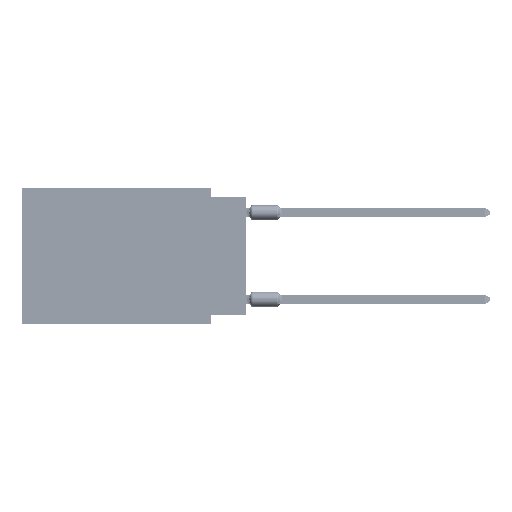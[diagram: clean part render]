
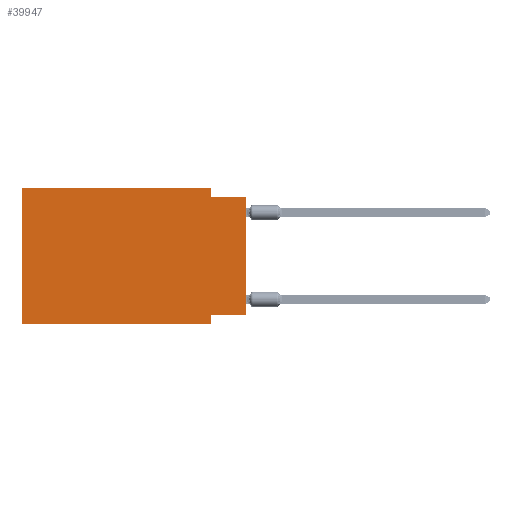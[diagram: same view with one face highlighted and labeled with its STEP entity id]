
A CAD part, left-side view. The second image highlights one B-rep face of the part: STEP entity #39947.
In plain terms, the highlighted planar face has unit normal (-1, 0, 0).
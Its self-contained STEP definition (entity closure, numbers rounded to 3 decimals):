
#1389 = ORIENTED_EDGE ( 'NONE', *, *, #11640, .F. ) ;
#4130 = ORIENTED_EDGE ( 'NONE', *, *, #25909, .F. ) ;
#4822 = CARTESIAN_POINT ( 'NONE',  ( 0., 16.383, 0. ) ) ;
#5756 = CARTESIAN_POINT ( 'NONE',  ( 0., 2.54, 0. ) ) ;
#6396 = DIRECTION ( 'NONE',  ( 0., 0., -1. ) ) ;
#7795 = PLANE ( 'NONE',  #74138 ) ;
#8201 = LINE ( 'NONE', #14792, #29444 ) ;
#9254 = EDGE_CURVE ( 'NONE', #75738, #48889, #11334, .T. ) ;
#9797 = DIRECTION ( 'NONE',  ( 0., 1., 0. ) ) ;
#9805 = DIRECTION ( 'NONE',  ( 0., 0., 1. ) ) ;
#11334 = LINE ( 'NONE', #55531, #68554 ) ;
#11640 = EDGE_CURVE ( 'NONE', #41968, #43702, #8201, .T. ) ;
#12406 = EDGE_CURVE ( 'NONE', #75738, #51605, #61400, .T. ) ;
#13184 = LINE ( 'NONE', #18564, #60067 ) ;
#14188 = VERTEX_POINT ( 'NONE', #55152 ) ;
#14792 = CARTESIAN_POINT ( 'NONE',  ( 0., 0., -0.635 ) ) ;
#15483 = EDGE_CURVE ( 'NONE', #23497, #41968, #19170, .T. ) ;
#18564 = CARTESIAN_POINT ( 'NONE',  ( 0., 2.54, -9.906 ) ) ;
#18953 = CARTESIAN_POINT ( 'NONE',  ( 0., 16.383, 0. ) ) ;
#19170 = LINE ( 'NONE', #31602, #31689 ) ;
#23497 = VERTEX_POINT ( 'NONE', #5756 ) ;
#24033 = CARTESIAN_POINT ( 'NONE',  ( 0., 2.54, -0.635 ) ) ;
#25183 = DIRECTION ( 'NONE',  ( 0., 0., -1. ) ) ;
#25909 = EDGE_CURVE ( 'NONE', #14188, #46694, #59363, .T. ) ;
#28476 = CARTESIAN_POINT ( 'NONE',  ( 0., 16.383, 0. ) ) ;
#29444 = VECTOR ( 'NONE', #40006, 1000. ) ;
#31602 = CARTESIAN_POINT ( 'NONE',  ( 0., 2.54, 0. ) ) ;
#31689 = VECTOR ( 'NONE', #6396, 1000. ) ;
#31906 = ORIENTED_EDGE ( 'NONE', *, *, #15483, .F. ) ;
#38205 = ORIENTED_EDGE ( 'NONE', *, *, #12406, .F. ) ;
#38868 = ORIENTED_EDGE ( 'NONE', *, *, #77032, .T. ) ;
#39947 = ADVANCED_FACE ( 'NONE', ( #45380 ), #7795, .F. ) ;
#40006 = DIRECTION ( 'NONE',  ( 0., -1., 0. ) ) ;
#41968 = VERTEX_POINT ( 'NONE', #24033 ) ;
#41993 = DIRECTION ( 'NONE',  ( 0., 0., 1. ) ) ;
#43136 = DIRECTION ( 'NONE',  ( 0., -1., 0. ) ) ;
#43702 = VERTEX_POINT ( 'NONE', #61495 ) ;
#43880 = EDGE_LOOP ( 'NONE', ( #38868, #1389, #31906, #44320, #38205, #60717, #58414, #4130 ) ) ;
#44155 = DIRECTION ( 'NONE',  ( 0., 0., -1. ) ) ;
#44320 = ORIENTED_EDGE ( 'NONE', *, *, #60778, .F. ) ;
#45380 = FACE_OUTER_BOUND ( 'NONE', #43880, .T. ) ;
#46694 = VERTEX_POINT ( 'NONE', #54308 ) ;
#48578 = CARTESIAN_POINT ( 'NONE',  ( 0., 16.383, -9.906 ) ) ;
#48889 = VERTEX_POINT ( 'NONE', #69753 ) ;
#48945 = EDGE_CURVE ( 'NONE', #46694, #48889, #13184, .T. ) ;
#49914 = VECTOR ( 'NONE', #9797, 1000. ) ;
#51592 = DIRECTION ( 'NONE',  ( 1., 0., 0. ) ) ;
#51605 = VERTEX_POINT ( 'NONE', #68489 ) ;
#54308 = CARTESIAN_POINT ( 'NONE',  ( 0., 2.54, -9.271 ) ) ;
#54420 = CARTESIAN_POINT ( 'NONE',  ( 0., 0., -9.271 ) ) ;
#55152 = CARTESIAN_POINT ( 'NONE',  ( 0., 0., -9.271 ) ) ;
#55531 = CARTESIAN_POINT ( 'NONE',  ( 0., 16.383, -9.906 ) ) ;
#58236 = VECTOR ( 'NONE', #41993, 1000. ) ;
#58414 = ORIENTED_EDGE ( 'NONE', *, *, #48945, .F. ) ;
#59223 = VECTOR ( 'NONE', #9805, 1000. ) ;
#59363 = LINE ( 'NONE', #54420, #49914 ) ;
#60067 = VECTOR ( 'NONE', #25183, 1000. ) ;
#60256 = LINE ( 'NONE', #28476, #77759 ) ;
#60717 = ORIENTED_EDGE ( 'NONE', *, *, #9254, .T. ) ;
#60778 = EDGE_CURVE ( 'NONE', #51605, #23497, #60256, .T. ) ;
#61400 = LINE ( 'NONE', #4822, #59223 ) ;
#61495 = CARTESIAN_POINT ( 'NONE',  ( 0., 0., -0.635 ) ) ;
#65624 = DIRECTION ( 'NONE',  ( 0., -1., 0. ) ) ;
#68489 = CARTESIAN_POINT ( 'NONE',  ( 0., 16.383, 0. ) ) ;
#68554 = VECTOR ( 'NONE', #43136, 1000. ) ;
#69753 = CARTESIAN_POINT ( 'NONE',  ( 0., 2.54, -9.906 ) ) ;
#73339 = CARTESIAN_POINT ( 'NONE',  ( 0., 0., 0. ) ) ;
#74138 = AXIS2_PLACEMENT_3D ( 'NONE', #18953, #51592, #44155 ) ;
#75738 = VERTEX_POINT ( 'NONE', #48578 ) ;
#77032 = EDGE_CURVE ( 'NONE', #14188, #43702, #79562, .T. ) ;
#77759 = VECTOR ( 'NONE', #65624, 1000. ) ;
#79562 = LINE ( 'NONE', #73339, #58236 ) ;
